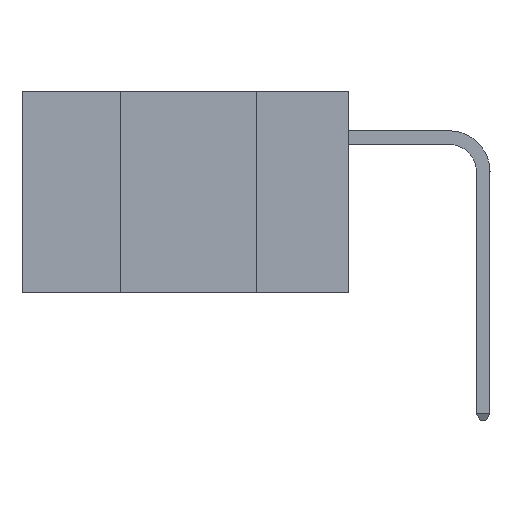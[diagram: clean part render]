
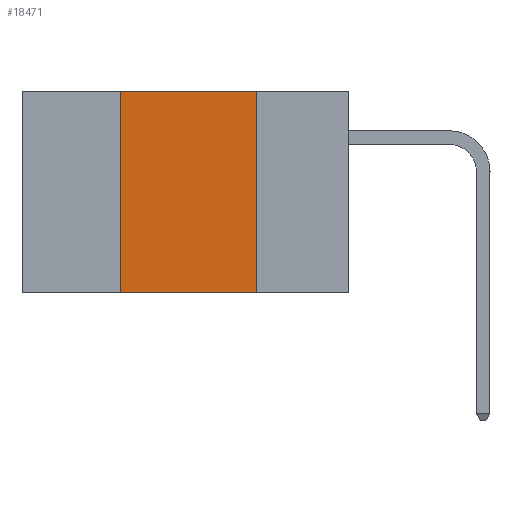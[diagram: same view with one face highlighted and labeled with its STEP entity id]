
A CAD part, left-side view. The second image highlights one B-rep face of the part: STEP entity #18471.
In plain terms, the highlighted planar face has unit normal (-1, 0, 0).
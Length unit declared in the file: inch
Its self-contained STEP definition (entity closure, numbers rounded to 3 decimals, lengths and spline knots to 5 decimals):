
#138 = DIRECTION ( 'NONE',  ( 0., -1., 0. ) ) ;
#1027 = EDGE_CURVE ( 'NONE', #23741, #26725, #34139, .T. ) ;
#2143 = VERTEX_POINT ( 'NONE', #16679 ) ;
#3044 = DIRECTION ( 'NONE',  ( 0., 0., -1. ) ) ;
#3290 = VECTOR ( 'NONE', #9409, 39.37008 ) ;
#3611 = VECTOR ( 'NONE', #31648, 39.37008 ) ;
#5536 = VERTEX_POINT ( 'NONE', #35808 ) ;
#9409 = DIRECTION ( 'NONE',  ( 0., 0., 1. ) ) ;
#11788 = CARTESIAN_POINT ( 'NONE',  ( 0., 0.17, -0.37 ) ) ;
#14100 = VECTOR ( 'NONE', #138, 39.37008 ) ;
#14199 = CARTESIAN_POINT ( 'NONE',  ( 0., 0.6, 0. ) ) ;
#14211 = EDGE_CURVE ( 'NONE', #5536, #2143, #25573, .T. ) ;
#15191 = AXIS2_PLACEMENT_3D ( 'NONE', #14199, #19822, #3044 ) ;
#16427 = DIRECTION ( 'NONE',  ( 0., -1., 0. ) ) ;
#16679 = CARTESIAN_POINT ( 'NONE',  ( 0., 0.42, 0. ) ) ;
#17699 = CARTESIAN_POINT ( 'NONE',  ( 0., 0.17, 0. ) ) ;
#18471 = ADVANCED_FACE ( 'NONE', ( #27761 ), #25259, .F. ) ;
#19822 = DIRECTION ( 'NONE',  ( 1., 0., 0. ) ) ;
#20697 = EDGE_LOOP ( 'NONE', ( #22573, #24016, #25322, #22871 ) ) ;
#21307 = CARTESIAN_POINT ( 'NONE',  ( 0., 0.17, 0. ) ) ;
#21543 = LINE ( 'NONE', #22524, #14100 ) ;
#21759 = EDGE_CURVE ( 'NONE', #5536, #26725, #21543, .T. ) ;
#21923 = CARTESIAN_POINT ( 'NONE',  ( 0., 0.6, 0. ) ) ;
#22524 = CARTESIAN_POINT ( 'NONE',  ( 0., 0.6, -0.37 ) ) ;
#22573 = ORIENTED_EDGE ( 'NONE', *, *, #1027, .F. ) ;
#22871 = ORIENTED_EDGE ( 'NONE', *, *, #21759, .T. ) ;
#23741 = VERTEX_POINT ( 'NONE', #21307 ) ;
#24016 = ORIENTED_EDGE ( 'NONE', *, *, #32304, .F. ) ;
#25155 = VECTOR ( 'NONE', #16427, 39.37008 ) ;
#25259 = PLANE ( 'NONE',  #15191 ) ;
#25322 = ORIENTED_EDGE ( 'NONE', *, *, #14211, .F. ) ;
#25573 = LINE ( 'NONE', #26140, #3290 ) ;
#26140 = CARTESIAN_POINT ( 'NONE',  ( 0., 0.42, 0. ) ) ;
#26725 = VERTEX_POINT ( 'NONE', #11788 ) ;
#27761 = FACE_OUTER_BOUND ( 'NONE', #20697, .T. ) ;
#31648 = DIRECTION ( 'NONE',  ( 0., 0., -1. ) ) ;
#32304 = EDGE_CURVE ( 'NONE', #2143, #23741, #33414, .T. ) ;
#33414 = LINE ( 'NONE', #21923, #25155 ) ;
#34139 = LINE ( 'NONE', #17699, #3611 ) ;
#35808 = CARTESIAN_POINT ( 'NONE',  ( 0., 0.42, -0.37 ) ) ;
